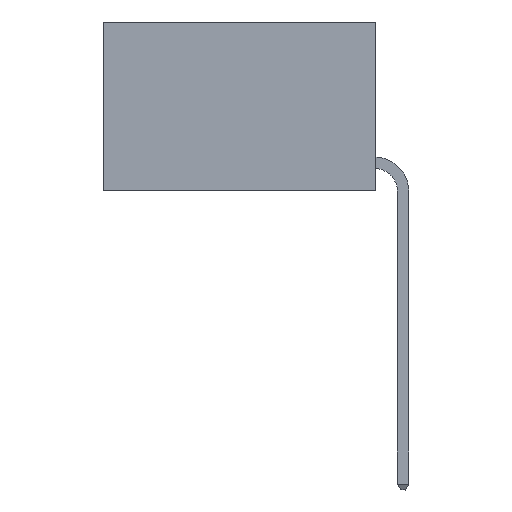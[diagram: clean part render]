
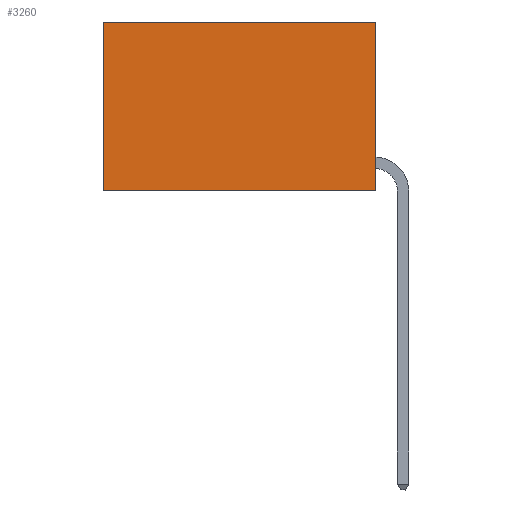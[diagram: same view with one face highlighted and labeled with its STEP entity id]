
A CAD part, left-side view. The second image highlights one B-rep face of the part: STEP entity #3260.
In plain terms, the highlighted planar face has unit normal (-1, 0, 0).
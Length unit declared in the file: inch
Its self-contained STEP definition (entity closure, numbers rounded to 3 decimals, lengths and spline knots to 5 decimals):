
#333 = VECTOR ( 'NONE', #3118, 39.37008 ) ;
#809 = CARTESIAN_POINT ( 'NONE',  ( 0.2625, 0., 0. ) ) ;
#1116 = VERTEX_POINT ( 'NONE', #13917 ) ;
#2384 = CARTESIAN_POINT ( 'NONE',  ( 0.2625, 0., 0. ) ) ;
#2462 = EDGE_CURVE ( 'NONE', #5000, #11592, #9716, .T. ) ;
#2672 = EDGE_CURVE ( 'NONE', #5000, #14652, #14051, .T. ) ;
#3118 = DIRECTION ( 'NONE',  ( 0., 1., 0. ) ) ;
#3196 = LINE ( 'NONE', #6562, #14317 ) ;
#3251 = FACE_OUTER_BOUND ( 'NONE', #3755, .T. ) ;
#3260 = ADVANCED_FACE ( 'NONE', ( #3251 ), #6971, .F. ) ;
#3449 = VECTOR ( 'NONE', #6491, 39.37008 ) ;
#3648 = DIRECTION ( 'NONE',  ( 1., 0., 0. ) ) ;
#3755 = EDGE_LOOP ( 'NONE', ( #12314, #3840, #14645, #10745 ) ) ;
#3840 = ORIENTED_EDGE ( 'NONE', *, *, #13070, .F. ) ;
#5000 = VERTEX_POINT ( 'NONE', #13615 ) ;
#5242 = VECTOR ( 'NONE', #9106, 39.37008 ) ;
#5593 = CARTESIAN_POINT ( 'NONE',  ( 0.2625, 0.6, 0. ) ) ;
#6491 = DIRECTION ( 'NONE',  ( 0., 1., 0. ) ) ;
#6562 = CARTESIAN_POINT ( 'NONE',  ( 0.2625, 0.6, 0. ) ) ;
#6971 = PLANE ( 'NONE',  #9101 ) ;
#7670 = DIRECTION ( 'NONE',  ( 0., 0., -1. ) ) ;
#8671 = CARTESIAN_POINT ( 'NONE',  ( 0.2625, 0., -0.37 ) ) ;
#9101 = AXIS2_PLACEMENT_3D ( 'NONE', #11806, #3648, #11433 ) ;
#9106 = DIRECTION ( 'NONE',  ( 0., 0., -1. ) ) ;
#9115 = CARTESIAN_POINT ( 'NONE',  ( 0.2625, 0., -0.37 ) ) ;
#9716 = LINE ( 'NONE', #809, #3449 ) ;
#10745 = ORIENTED_EDGE ( 'NONE', *, *, #2462, .T. ) ;
#11433 = DIRECTION ( 'NONE',  ( 0., 0., -1. ) ) ;
#11592 = VERTEX_POINT ( 'NONE', #5593 ) ;
#11806 = CARTESIAN_POINT ( 'NONE',  ( 0.2625, 0., 0. ) ) ;
#12314 = ORIENTED_EDGE ( 'NONE', *, *, #13123, .T. ) ;
#12440 = LINE ( 'NONE', #8671, #333 ) ;
#13070 = EDGE_CURVE ( 'NONE', #14652, #1116, #12440, .T. ) ;
#13123 = EDGE_CURVE ( 'NONE', #11592, #1116, #3196, .T. ) ;
#13615 = CARTESIAN_POINT ( 'NONE',  ( 0.2625, 0., 0. ) ) ;
#13917 = CARTESIAN_POINT ( 'NONE',  ( 0.2625, 0.6, -0.37 ) ) ;
#14051 = LINE ( 'NONE', #2384, #5242 ) ;
#14317 = VECTOR ( 'NONE', #7670, 39.37008 ) ;
#14645 = ORIENTED_EDGE ( 'NONE', *, *, #2672, .F. ) ;
#14652 = VERTEX_POINT ( 'NONE', #9115 ) ;
